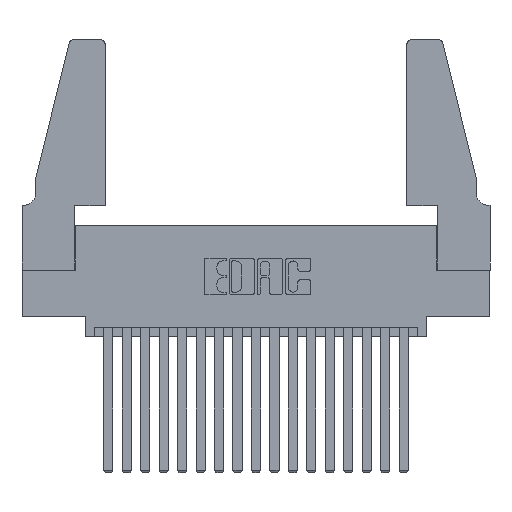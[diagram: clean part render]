
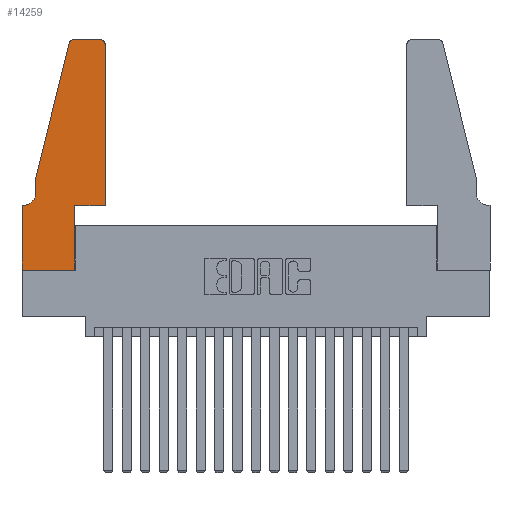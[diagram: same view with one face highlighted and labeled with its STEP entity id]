
A CAD part, top view. The second image highlights one B-rep face of the part: STEP entity #14259.
In plain terms, the highlighted planar face has unit normal (0, 0, 1).
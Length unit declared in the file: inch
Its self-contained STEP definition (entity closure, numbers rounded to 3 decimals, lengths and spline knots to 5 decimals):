
#82 = VECTOR ( 'NONE', #4881, 39.37008 ) ;
#84 = CARTESIAN_POINT ( 'NONE',  ( 0.4205, 1.22, 0.37 ) ) ;
#140 = VERTEX_POINT ( 'NONE', #1980 ) ;
#292 = AXIS2_PLACEMENT_3D ( 'NONE', #9878, #1078, #11353 ) ;
#379 = DIRECTION ( 'NONE',  ( 0., 0., 1. ) ) ;
#442 = CARTESIAN_POINT ( 'NONE',  ( 0.0755, 0.35, 0.37 ) ) ;
#789 = LINE ( 'NONE', #18275, #8157 ) ;
#882 = VERTEX_POINT ( 'NONE', #1422 ) ;
#887 = DIRECTION ( 'NONE',  ( 0., -1., 0. ) ) ;
#996 = CARTESIAN_POINT ( 'NONE',  ( 0.4505, 0.35, 0.37 ) ) ;
#1078 = DIRECTION ( 'NONE',  ( 0., 0., -1. ) ) ;
#1249 = DIRECTION ( 'NONE',  ( 0., 0., 1. ) ) ;
#1326 = CIRCLE ( 'NONE', #292, 0.07 ) ;
#1422 = CARTESIAN_POINT ( 'NONE',  ( 0., 0.35, 0.37 ) ) ;
#1622 = DIRECTION ( 'NONE',  ( 1., 0., 0. ) ) ;
#1980 = CARTESIAN_POINT ( 'NONE',  ( 0.4505, 0.35, 0.37 ) ) ;
#2373 = EDGE_CURVE ( 'NONE', #11826, #13179, #18128, .T. ) ;
#2386 = EDGE_CURVE ( 'NONE', #13179, #140, #2745, .T. ) ;
#2633 = DIRECTION ( 'NONE',  ( -0.239, -0.971, 0. ) ) ;
#2725 = LINE ( 'NONE', #9071, #17679 ) ;
#2745 = LINE ( 'NONE', #7361, #10083 ) ;
#2859 = EDGE_CURVE ( 'NONE', #10516, #11826, #2725, .T. ) ;
#3216 = LINE ( 'NONE', #3969, #6634 ) ;
#3322 = CARTESIAN_POINT ( 'NONE',  ( 0.2605, 1.25, 0.37 ) ) ;
#3969 = CARTESIAN_POINT ( 'NONE',  ( 0.0755, 0.5, 0.37 ) ) ;
#4289 = CARTESIAN_POINT ( 'NONE',  ( 0.0055, 0.35, 0.37 ) ) ;
#4881 = DIRECTION ( 'NONE',  ( -1., 0., 0. ) ) ;
#5338 = CARTESIAN_POINT ( 'NONE',  ( 0.4505, 1.22, 0.37 ) ) ;
#5625 = CARTESIAN_POINT ( 'NONE',  ( 0.2865, 0., 0.37 ) ) ;
#5661 = PLANE ( 'NONE',  #10983 ) ;
#5998 = VECTOR ( 'NONE', #2633, 39.37008 ) ;
#6358 = AXIS2_PLACEMENT_3D ( 'NONE', #9191, #379, #10672 ) ;
#6634 = VECTOR ( 'NONE', #18406, 39.37008 ) ;
#6639 = VECTOR ( 'NONE', #11647, 39.37008 ) ;
#6871 = CIRCLE ( 'NONE', #6358, 0.03 ) ;
#6919 = DIRECTION ( 'NONE',  ( 0., 1., 0. ) ) ;
#7178 = EDGE_CURVE ( 'NONE', #9794, #7252, #17508, .T. ) ;
#7252 = VERTEX_POINT ( 'NONE', #18645 ) ;
#7253 = ORIENTED_EDGE ( 'NONE', *, *, #14992, .T. ) ;
#7310 = ORIENTED_EDGE ( 'NONE', *, *, #18005, .T. ) ;
#7348 = DIRECTION ( 'NONE',  ( 1., 0., 0. ) ) ;
#7361 = CARTESIAN_POINT ( 'NONE',  ( 0.4505, 0.35, 0.37 ) ) ;
#7501 = ORIENTED_EDGE ( 'NONE', *, *, #17472, .T. ) ;
#7573 = VERTEX_POINT ( 'NONE', #15140 ) ;
#7600 = LINE ( 'NONE', #3322, #11056 ) ;
#7759 = ORIENTED_EDGE ( 'NONE', *, *, #7178, .T. ) ;
#7786 = DIRECTION ( 'NONE',  ( 1., 0., 0. ) ) ;
#7936 = VECTOR ( 'NONE', #6919, 39.37008 ) ;
#8109 = ORIENTED_EDGE ( 'NONE', *, *, #17237, .T. ) ;
#8125 = ORIENTED_EDGE ( 'NONE', *, *, #9536, .T. ) ;
#8157 = VECTOR ( 'NONE', #887, 39.37008 ) ;
#8233 = ORIENTED_EDGE ( 'NONE', *, *, #9758, .T. ) ;
#8336 = ORIENTED_EDGE ( 'NONE', *, *, #2859, .T. ) ;
#8339 = VERTEX_POINT ( 'NONE', #13943 ) ;
#8350 = ORIENTED_EDGE ( 'NONE', *, *, #2373, .T. ) ;
#8458 = ORIENTED_EDGE ( 'NONE', *, *, #2386, .T. ) ;
#8474 = ORIENTED_EDGE ( 'NONE', *, *, #10368, .T. ) ;
#9023 = ORIENTED_EDGE ( 'NONE', *, *, #9970, .T. ) ;
#9071 = CARTESIAN_POINT ( 'NONE',  ( 0., 0., 0.37 ) ) ;
#9182 = DIRECTION ( 'NONE',  ( -1., 0., 0. ) ) ;
#9191 = CARTESIAN_POINT ( 'NONE',  ( 0.284, 1.22, 0.37 ) ) ;
#9536 = EDGE_CURVE ( 'NONE', #11844, #882, #15635, .T. ) ;
#9751 = CARTESIAN_POINT ( 'NONE',  ( 0.25487, 1.22718, 0.37 ) ) ;
#9758 = EDGE_CURVE ( 'NONE', #882, #10516, #789, .T. ) ;
#9794 = VERTEX_POINT ( 'NONE', #9751 ) ;
#9878 = CARTESIAN_POINT ( 'NONE',  ( 0.0055, 0.42, 0.37 ) ) ;
#9970 = EDGE_CURVE ( 'NONE', #10971, #7573, #16063, .T. ) ;
#10006 = LINE ( 'NONE', #996, #7936 ) ;
#10049 = CARTESIAN_POINT ( 'NONE',  ( 0., 0.35, 0.37 ) ) ;
#10083 = VECTOR ( 'NONE', #7348, 39.37008 ) ;
#10368 = EDGE_CURVE ( 'NONE', #140, #10971, #10006, .T. ) ;
#10398 = DIRECTION ( 'NONE',  ( 0., 0., 1. ) ) ;
#10516 = VERTEX_POINT ( 'NONE', #14529 ) ;
#10672 = DIRECTION ( 'NONE',  ( 1., 0., 0. ) ) ;
#10971 = VERTEX_POINT ( 'NONE', #5338 ) ;
#10983 = AXIS2_PLACEMENT_3D ( 'NONE', #10049, #1249, #11526 ) ;
#11056 = VECTOR ( 'NONE', #9182, 39.37008 ) ;
#11253 = CARTESIAN_POINT ( 'NONE',  ( 0.2865, 0.35, 0.37 ) ) ;
#11353 = DIRECTION ( 'NONE',  ( -1., 0., 0. ) ) ;
#11526 = DIRECTION ( 'NONE',  ( 1., 0., 0. ) ) ;
#11647 = DIRECTION ( 'NONE',  ( 0., 1., 0. ) ) ;
#11826 = VERTEX_POINT ( 'NONE', #5625 ) ;
#11844 = VERTEX_POINT ( 'NONE', #4289 ) ;
#12026 = EDGE_LOOP ( 'NONE', ( #7253, #8109, #7759, #7501, #7310, #8125, #8233, #8336, #8350, #8458, #8474, #9023 ) ) ;
#12883 = CARTESIAN_POINT ( 'NONE',  ( 0.0755, 0.5, 0.37 ) ) ;
#13179 = VERTEX_POINT ( 'NONE', #14868 ) ;
#13833 = VERTEX_POINT ( 'NONE', #16353 ) ;
#13943 = CARTESIAN_POINT ( 'NONE',  ( 0.284, 1.25, 0.37 ) ) ;
#14259 = ADVANCED_FACE ( 'NONE', ( #18447 ), #5661, .T. ) ;
#14529 = CARTESIAN_POINT ( 'NONE',  ( 0., 0., 0.37 ) ) ;
#14868 = CARTESIAN_POINT ( 'NONE',  ( 0.2865, 0.35, 0.37 ) ) ;
#14992 = EDGE_CURVE ( 'NONE', #7573, #8339, #7600, .T. ) ;
#15140 = CARTESIAN_POINT ( 'NONE',  ( 0.4205, 1.25, 0.37 ) ) ;
#15635 = LINE ( 'NONE', #442, #82 ) ;
#16063 = CIRCLE ( 'NONE', #16681, 0.03 ) ;
#16353 = CARTESIAN_POINT ( 'NONE',  ( 0.0755, 0.42, 0.37 ) ) ;
#16681 = AXIS2_PLACEMENT_3D ( 'NONE', #84, #10398, #1622 ) ;
#17237 = EDGE_CURVE ( 'NONE', #8339, #9794, #6871, .T. ) ;
#17472 = EDGE_CURVE ( 'NONE', #7252, #13833, #3216, .T. ) ;
#17508 = LINE ( 'NONE', #12883, #5998 ) ;
#17679 = VECTOR ( 'NONE', #7786, 39.37008 ) ;
#18005 = EDGE_CURVE ( 'NONE', #13833, #11844, #1326, .T. ) ;
#18128 = LINE ( 'NONE', #11253, #6639 ) ;
#18275 = CARTESIAN_POINT ( 'NONE',  ( 0., 0., 0.37 ) ) ;
#18406 = DIRECTION ( 'NONE',  ( 0., -1., 0. ) ) ;
#18447 = FACE_OUTER_BOUND ( 'NONE', #12026, .T. ) ;
#18645 = CARTESIAN_POINT ( 'NONE',  ( 0.0755, 0.5, 0.37 ) ) ;
